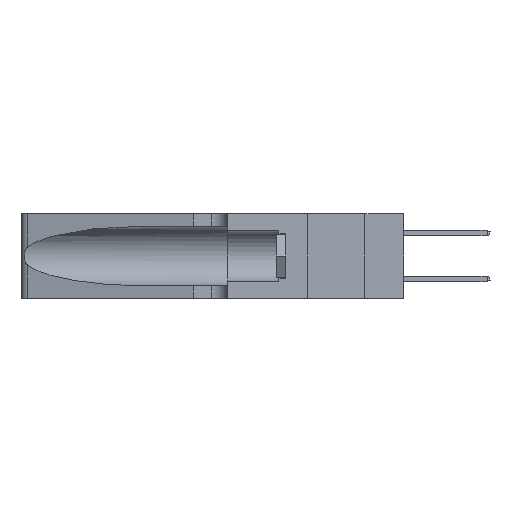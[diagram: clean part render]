
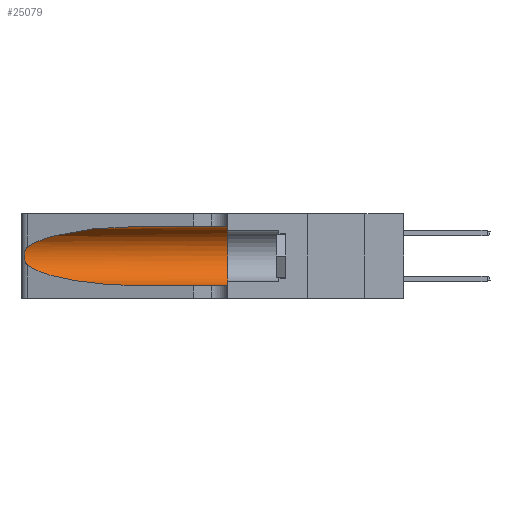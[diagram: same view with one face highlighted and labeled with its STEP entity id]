
A CAD part, left-side view. The second image highlights one B-rep face of the part: STEP entity #25079.
In plain terms, the highlighted cylindrical face has radius 3.308 mm (diameter 6.617 mm), a partial arc.
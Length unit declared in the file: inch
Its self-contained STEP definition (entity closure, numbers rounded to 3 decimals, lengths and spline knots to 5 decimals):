
#163 = CARTESIAN_POINT ( 'NONE',  ( 0.1305, 0.72297, 0.05475 ) ) ;
#745 = CARTESIAN_POINT ( 'NONE',  ( 0.25639, 1.23186, 0.15144 ) ) ;
#2638 = CARTESIAN_POINT ( 'NONE',  ( 0.25487, 1.22718, 0.14631 ) ) ;
#3326 = CARTESIAN_POINT ( 'NONE',  ( 0.25487, 1.22718, 0.14631 ) ) ;
#3677 = EDGE_CURVE ( 'NONE', #4036, #13919, #30271, .T. ) ;
#4036 = VERTEX_POINT ( 'NONE', #10563 ) ;
#4370 = DIRECTION ( 'NONE',  ( 0., 1., 0. ) ) ;
#4748 = ORIENTED_EDGE ( 'NONE', *, *, #22025, .F. ) ;
#4852 = CARTESIAN_POINT ( 'NONE',  ( 0.1305, 1.61858, 0.31525 ) ) ;
#4992 = B_SPLINE_CURVE_WITH_KNOTS ( 'NONE', 3,
 ( #13260, #18187, #5778, #23069, #8290, #25507, #10814, #27952, #13366, #30408, #15835, #745, #18297, #3326 ),
 .UNSPECIFIED., .F., .F.,
 ( 4, 2, 2, 2, 2, 2, 4 ),
 ( 0., 0.00027, 0.00053, 0.00107, 0.0016, 0.00187, 0.00214 ),
 .UNSPECIFIED. ) ;
#5548 = VERTEX_POINT ( 'NONE', #28955 ) ;
#5778 = CARTESIAN_POINT ( 'NONE',  ( 0.25639, 1.23184, 0.21858 ) ) ;
#6369 = CARTESIAN_POINT ( 'NONE',  ( 0.1305, 0.35, 0.05475 ) ) ;
#6978 = CYLINDRICAL_SURFACE ( 'NONE', #22299, 0.13025 ) ;
#7792 = FACE_OUTER_BOUND ( 'NONE', #20215, .T. ) ;
#8290 = CARTESIAN_POINT ( 'NONE',  ( 0.25854, 1.2359, 0.20912 ) ) ;
#8937 = VERTEX_POINT ( 'NONE', #14156 ) ;
#9221 = CARTESIAN_POINT ( 'NONE',  ( 0.1305, 1.61858, 0.05475 ) ) ;
#10563 = CARTESIAN_POINT ( 'NONE',  ( 0.1305, 0.72297, 0.31525 ) ) ;
#10699 = CARTESIAN_POINT ( 'NONE',  ( 0.1305, 0.35, 0.31525 ) ) ;
#10793 = VERTEX_POINT ( 'NONE', #6369 ) ;
#10814 = CARTESIAN_POINT ( 'NONE',  ( 0.26075, 1.23896, 0.19203 ) ) ;
#10837 =( BOUNDED_CURVE ( )  B_SPLINE_CURVE ( 3, ( #2638, #27398, #15298, #163 ),
 .UNSPECIFIED., .F., .T. ) 
 B_SPLINE_CURVE_WITH_KNOTS ( ( 4, 4 ),
 ( 3.44316, 4.71239 ),
 .UNSPECIFIED. ) 
 CURVE ( )  GEOMETRIC_REPRESENTATION_ITEM ( )  RATIONAL_B_SPLINE_CURVE ( ( 1., 0.87, 0.87, 1. ) ) 
 REPRESENTATION_ITEM ( '' )  );
#11440 = ORIENTED_EDGE ( 'NONE', *, *, #22126, .T. ) ;
#12041 = ORIENTED_EDGE ( 'NONE', *, *, #3677, .T. ) ;
#13260 = CARTESIAN_POINT ( 'NONE',  ( 0.25487, 1.22718, 0.22369 ) ) ;
#13366 = CARTESIAN_POINT ( 'NONE',  ( 0.26017, 1.23833, 0.17102 ) ) ;
#13626 = ORIENTED_EDGE ( 'NONE', *, *, #23571, .T. ) ;
#13716 = VERTEX_POINT ( 'NONE', #10699 ) ;
#13919 = VERTEX_POINT ( 'NONE', #26637 ) ;
#14156 = CARTESIAN_POINT ( 'NONE',  ( 0.1305, 0.72297, 0.05475 ) ) ;
#14212 = CARTESIAN_POINT ( 'NONE',  ( 0.18966, 0.96281, 0.31525 ) ) ;
#14854 = DIRECTION ( 'NONE',  ( 0., 0., -1. ) ) ;
#14863 = DIRECTION ( 'NONE',  ( 0., -1., 0. ) ) ;
#15298 = CARTESIAN_POINT ( 'NONE',  ( 0.18966, 0.96281, 0.05475 ) ) ;
#15835 = CARTESIAN_POINT ( 'NONE',  ( 0.25789, 1.23486, 0.15765 ) ) ;
#16677 = CARTESIAN_POINT ( 'NONE',  ( 0.1305, 0.72297, 0.31525 ) ) ;
#18187 = CARTESIAN_POINT ( 'NONE',  ( 0.25555, 1.22994, 0.2215 ) ) ;
#18297 = CARTESIAN_POINT ( 'NONE',  ( 0.25555, 1.22993, 0.14849 ) ) ;
#19129 = CARTESIAN_POINT ( 'NONE',  ( 0.25487, 1.22718, 0.22369 ) ) ;
#19316 = CARTESIAN_POINT ( 'NONE',  ( 0.1305, 0.35, 0.185 ) ) ;
#20215 = EDGE_LOOP ( 'NONE', ( #12041, #13626, #11440, #27886, #23380, #4748 ) ) ;
#20644 = EDGE_CURVE ( 'NONE', #8937, #10793, #28425, .T. ) ;
#21759 = DIRECTION ( 'NONE',  ( 0., 0., 1. ) ) ;
#22025 = EDGE_CURVE ( 'NONE', #4036, #13716, #27621, .T. ) ;
#22126 = EDGE_CURVE ( 'NONE', #5548, #8937, #10837, .T. ) ;
#22299 = AXIS2_PLACEMENT_3D ( 'NONE', #29431, #31839, #14854 ) ;
#22594 = CIRCLE ( 'NONE', #31007, 0.13025 ) ;
#23069 = CARTESIAN_POINT ( 'NONE',  ( 0.25787, 1.23484, 0.2124 ) ) ;
#23380 = ORIENTED_EDGE ( 'NONE', *, *, #30081, .F. ) ;
#23571 = EDGE_CURVE ( 'NONE', #13919, #5548, #4992, .T. ) ;
#23949 = DIRECTION ( 'NONE',  ( 0., -1., 0. ) ) ;
#25079 = ADVANCED_FACE ( 'NONE', ( #7792 ), #6978, .F. ) ;
#25507 = CARTESIAN_POINT ( 'NONE',  ( 0.26018, 1.23835, 0.19895 ) ) ;
#26637 = CARTESIAN_POINT ( 'NONE',  ( 0.25487, 1.22718, 0.22369 ) ) ;
#26837 = VECTOR ( 'NONE', #14863, 39.37008 ) ;
#27398 = CARTESIAN_POINT ( 'NONE',  ( 0.2373, 1.15595, 0.08982 ) ) ;
#27621 = LINE ( 'NONE', #4852, #26837 ) ;
#27668 = VECTOR ( 'NONE', #23949, 39.37008 ) ;
#27886 = ORIENTED_EDGE ( 'NONE', *, *, #20644, .T. ) ;
#27952 = CARTESIAN_POINT ( 'NONE',  ( 0.26075, 1.23896, 0.178 ) ) ;
#28425 = LINE ( 'NONE', #9221, #27668 ) ;
#28784 = CARTESIAN_POINT ( 'NONE',  ( 0.2373, 1.15595, 0.28018 ) ) ;
#28955 = CARTESIAN_POINT ( 'NONE',  ( 0.25487, 1.22718, 0.14631 ) ) ;
#29431 = CARTESIAN_POINT ( 'NONE',  ( 0.1305, 1.61858, 0.185 ) ) ;
#30081 = EDGE_CURVE ( 'NONE', #13716, #10793, #22594, .T. ) ;
#30271 =( BOUNDED_CURVE ( )  B_SPLINE_CURVE ( 3, ( #16677, #14212, #28784, #19129 ),
 .UNSPECIFIED., .F., .F. ) 
 B_SPLINE_CURVE_WITH_KNOTS ( ( 4, 4 ),
 ( 1.5708, 2.84003 ),
 .UNSPECIFIED. ) 
 CURVE ( )  GEOMETRIC_REPRESENTATION_ITEM ( )  RATIONAL_B_SPLINE_CURVE ( ( 1., 0.87, 0.87, 1. ) ) 
 REPRESENTATION_ITEM ( '' )  );
#30408 = CARTESIAN_POINT ( 'NONE',  ( 0.25856, 1.23593, 0.16098 ) ) ;
#31007 = AXIS2_PLACEMENT_3D ( 'NONE', #19316, #4370, #21759 ) ;
#31839 = DIRECTION ( 'NONE',  ( 0., -1., 0. ) ) ;
